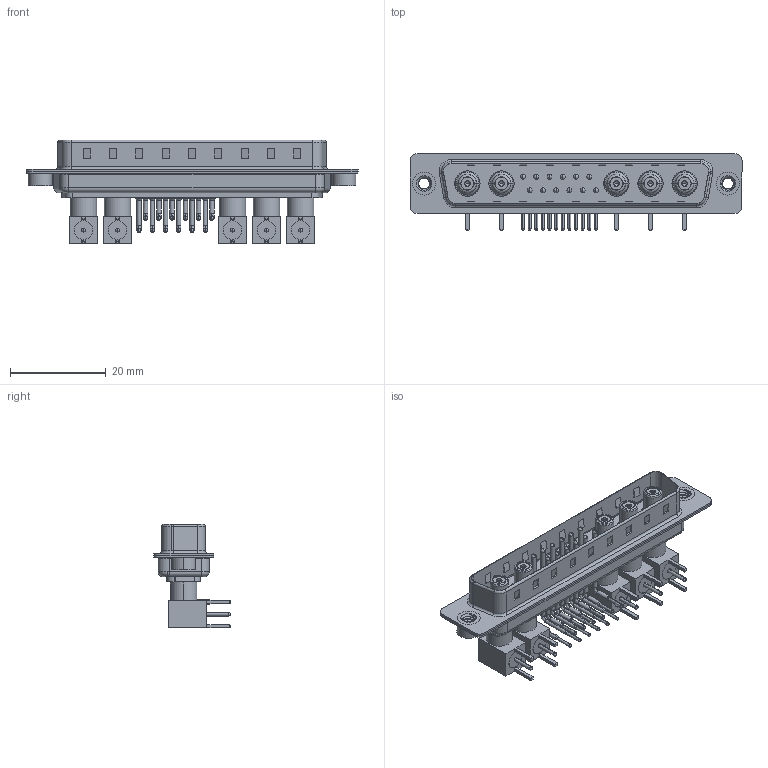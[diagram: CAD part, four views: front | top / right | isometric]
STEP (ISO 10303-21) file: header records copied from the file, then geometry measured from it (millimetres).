
FILE_DESCRIPTION (( 'STEP AP203' ), '1' );
FILE_NAME ('629-17W5640-7NA.STEP', '2022-05-16T00:47:05', ( '' ), ( '' ), 'SwSTEP 2.0', 'SolidWorks 2020', '' );
FILE_SCHEMA (( 'CONFIG_CONTROL_DESIGN' ));
Length unit declared in the file: millimetre
Products named in the file (19): 629Combo Shell Rear_37 Contacts; 629-17W5640-7NA; Locking Collar; Socket_RA; RA Back Shell; 629Combo Shell Front_37 Contacts; Co-Ax Jack Assy_RA; Co-Ax Jack_RA PC Tail; 629Combo Contact Row 1; Insulator Socket; Insulator RA Pin; Insulator Socket 2; 629Combo Contact Row 2; 629Combo Threaded Rivet_2; 629Combo Housing_17W5
Assembly tree (57 placements, depth 3):
  629-17W5640-7NA
    629Combo Housing_17W5
    629Combo Shell Rear_37 Contacts
    629Combo Shell Front_37 Contacts
    629Combo Threaded Rivet_2  x2
    Co-Ax Jack Assy_RA
      Co-Ax Jack_RA PC Tail
      Insulator Socket
      Insulator Socket 2
      Locking Collar
      Socket_RA
      RA Back Shell
      Insulator RA Pin
    Co-Ax Jack Assy_RA
      Co-Ax Jack_RA PC Tail
      Insulator Socket
      Insulator Socket 2
      Locking Collar
      Socket_RA
      RA Back Shell
      Insulator RA Pin
    Co-Ax Jack Assy_RA
      Co-Ax Jack_RA PC Tail
      Insulator Socket
      Insulator Socket 2
      Locking Collar
      Socket_RA
      RA Back Shell
      Insulator RA Pin
    Co-Ax Jack Assy_RA
      Co-Ax Jack_RA PC Tail
      Insulator Socket
      Insulator Socket 2
      Locking Collar
      Socket_RA
      RA Back Shell
      Insulator RA Pin
    Co-Ax Jack Assy_RA
      Co-Ax Jack_RA PC Tail
      Insulator Socket
      Insulator Socket 2
      Locking Collar
      Socket_RA
      RA Back Shell
      Insulator RA Pin
    629Combo Contact Row 1  x6
    629Combo Contact Row 2  x6
Bounding box: 69.4 x 16 x 21.71 mm (x, y, z)
Volume: 5291.9 mm3; surface area: 14211.2 mm2
Topology: 52 solids, 52 shells, 2492 faces, 6514 edges, 4167 vertices
Faces by surface type: plane 1256, cylinder 908, cone 155, bspline 83, torus 80, sphere 10
Entity records: 30786 total; most frequent: CARTESIAN_POINT 6360, DIRECTION 4670, ORIENTED_EDGE 4302, EDGE_CURVE 2151, AXIS2_PLACEMENT_3D 1684, VERTEX_POINT 1383, LINE 1302, VECTOR 1302
